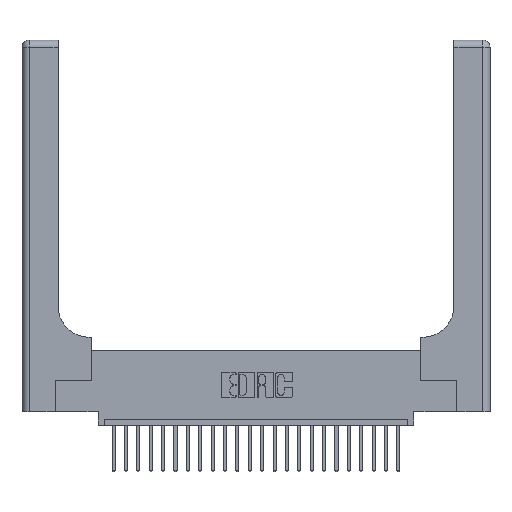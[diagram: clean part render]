
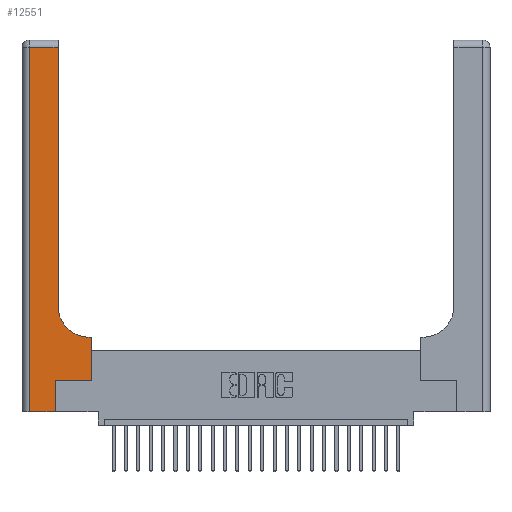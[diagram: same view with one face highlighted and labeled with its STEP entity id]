
A CAD part, top view. The second image highlights one B-rep face of the part: STEP entity #12551.
In plain terms, the highlighted planar face has unit normal (0, 0, 1).
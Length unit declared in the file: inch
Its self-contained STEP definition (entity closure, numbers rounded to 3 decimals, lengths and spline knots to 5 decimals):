
#106 = CARTESIAN_POINT ( 'NONE',  ( 0., 2.94, 0.37 ) ) ;
#196 = LINE ( 'NONE', #1382, #11151 ) ;
#1212 = EDGE_CURVE ( 'NONE', #1856, #20556, #21305, .T. ) ;
#1359 = ORIENTED_EDGE ( 'NONE', *, *, #15520, .T. ) ;
#1382 = CARTESIAN_POINT ( 'NONE',  ( 0., 0., 0.37 ) ) ;
#1856 = VERTEX_POINT ( 'NONE', #19534 ) ;
#2181 = VERTEX_POINT ( 'NONE', #15146 ) ;
#2373 = DIRECTION ( 'NONE',  ( -1., 0., 0. ) ) ;
#2596 = PLANE ( 'NONE',  #16368 ) ;
#3448 = EDGE_CURVE ( 'NONE', #17414, #22764, #19940, .T. ) ;
#3915 = LINE ( 'NONE', #106, #7043 ) ;
#5138 = ORIENTED_EDGE ( 'NONE', *, *, #19640, .T. ) ;
#5488 = DIRECTION ( 'NONE',  ( 1., 0., 0. ) ) ;
#6141 = CARTESIAN_POINT ( 'NONE',  ( 0.269, 0.25, 0.37 ) ) ;
#7043 = VECTOR ( 'NONE', #2373, 39.37008 ) ;
#7593 = DIRECTION ( 'NONE',  ( 1., 0., 0. ) ) ;
#7741 = VERTEX_POINT ( 'NONE', #16094 ) ;
#7775 = LINE ( 'NONE', #21201, #13114 ) ;
#8025 = EDGE_CURVE ( 'NONE', #21359, #1856, #20071, .T. ) ;
#8887 = EDGE_CURVE ( 'NONE', #7741, #2181, #10092, .T. ) ;
#10092 = LINE ( 'NONE', #21326, #16028 ) ;
#10170 = ORIENTED_EDGE ( 'NONE', *, *, #1212, .T. ) ;
#10438 = DIRECTION ( 'NONE',  ( 1., 0., 0. ) ) ;
#10575 = ORIENTED_EDGE ( 'NONE', *, *, #25153, .T. ) ;
#10852 = VERTEX_POINT ( 'NONE', #19851 ) ;
#11017 = VECTOR ( 'NONE', #15571, 39.37008 ) ;
#11151 = VECTOR ( 'NONE', #5488, 39.37008 ) ;
#11335 = CARTESIAN_POINT ( 'NONE',  ( 0.5585, 0.25, 0.37 ) ) ;
#11536 = CARTESIAN_POINT ( 'NONE',  ( 0.2915, 2.94, 0.37 ) ) ;
#11872 = CARTESIAN_POINT ( 'NONE',  ( 0.2915, 0.85, 0.37 ) ) ;
#12108 = CARTESIAN_POINT ( 'NONE',  ( 0.2915, 0.6, 0.37 ) ) ;
#12451 = VECTOR ( 'NONE', #16264, 39.37008 ) ;
#12551 = ADVANCED_FACE ( 'NONE', ( #18615 ), #2596, .F. ) ;
#12745 = EDGE_CURVE ( 'NONE', #2181, #21359, #196, .T. ) ;
#13114 = VECTOR ( 'NONE', #15277, 39.37008 ) ;
#13147 = AXIS2_PLACEMENT_3D ( 'NONE', #15517, #19513, #7593 ) ;
#13477 = ORIENTED_EDGE ( 'NONE', *, *, #17887, .T. ) ;
#13913 = EDGE_LOOP ( 'NONE', ( #5138, #13477, #14412, #24519, #14323, #10170, #10575, #1359, #14639 ) ) ;
#14195 = CARTESIAN_POINT ( 'NONE',  ( 0.269, 0., 0.37 ) ) ;
#14323 = ORIENTED_EDGE ( 'NONE', *, *, #8025, .T. ) ;
#14412 = ORIENTED_EDGE ( 'NONE', *, *, #8887, .T. ) ;
#14627 = CARTESIAN_POINT ( 'NONE',  ( 0., 3., 0.37 ) ) ;
#14639 = ORIENTED_EDGE ( 'NONE', *, *, #3448, .T. ) ;
#15146 = CARTESIAN_POINT ( 'NONE',  ( 0.06, 0., 0.37 ) ) ;
#15277 = DIRECTION ( 'NONE',  ( 0., 1., 0. ) ) ;
#15517 = CARTESIAN_POINT ( 'NONE',  ( 0.5415, 0.85, 0.37 ) ) ;
#15520 = EDGE_CURVE ( 'NONE', #10852, #17414, #25807, .T. ) ;
#15571 = DIRECTION ( 'NONE',  ( 0., 1., 0. ) ) ;
#16028 = VECTOR ( 'NONE', #17558, 39.37008 ) ;
#16094 = CARTESIAN_POINT ( 'NONE',  ( 0.06, 2.94, 0.37 ) ) ;
#16264 = DIRECTION ( 'NONE',  ( -1., 0., 0. ) ) ;
#16324 = VECTOR ( 'NONE', #10438, 39.37008 ) ;
#16368 = AXIS2_PLACEMENT_3D ( 'NONE', #14627, #16441, #20634 ) ;
#16441 = DIRECTION ( 'NONE',  ( 0., 0., -1. ) ) ;
#16909 = LINE ( 'NONE', #17827, #11017 ) ;
#17414 = VERTEX_POINT ( 'NONE', #20358 ) ;
#17558 = DIRECTION ( 'NONE',  ( 0., -1., 0. ) ) ;
#17827 = CARTESIAN_POINT ( 'NONE',  ( 0.2915, 3., 0.37 ) ) ;
#17887 = EDGE_CURVE ( 'NONE', #19982, #7741, #3915, .T. ) ;
#18189 = DIRECTION ( 'NONE',  ( 0., 1., 0. ) ) ;
#18615 = FACE_OUTER_BOUND ( 'NONE', #13913, .T. ) ;
#18839 = VECTOR ( 'NONE', #18189, 39.37008 ) ;
#19513 = DIRECTION ( 'NONE',  ( 0., 0., -1. ) ) ;
#19534 = CARTESIAN_POINT ( 'NONE',  ( 0.269, 0.25, 0.37 ) ) ;
#19640 = EDGE_CURVE ( 'NONE', #22764, #19982, #16909, .T. ) ;
#19851 = CARTESIAN_POINT ( 'NONE',  ( 0.5585, 0.6, 0.37 ) ) ;
#19940 = CIRCLE ( 'NONE', #13147, 0.25 ) ;
#19982 = VERTEX_POINT ( 'NONE', #11536 ) ;
#20071 = LINE ( 'NONE', #14195, #18839 ) ;
#20358 = CARTESIAN_POINT ( 'NONE',  ( 0.5415, 0.6, 0.37 ) ) ;
#20442 = CARTESIAN_POINT ( 'NONE',  ( 0.269, 0., 0.37 ) ) ;
#20556 = VERTEX_POINT ( 'NONE', #11335 ) ;
#20634 = DIRECTION ( 'NONE',  ( -1., 0., 0. ) ) ;
#21201 = CARTESIAN_POINT ( 'NONE',  ( 0.5585, 0.25, 0.37 ) ) ;
#21305 = LINE ( 'NONE', #6141, #16324 ) ;
#21326 = CARTESIAN_POINT ( 'NONE',  ( 0.06, 3., 0.37 ) ) ;
#21359 = VERTEX_POINT ( 'NONE', #20442 ) ;
#22764 = VERTEX_POINT ( 'NONE', #11872 ) ;
#24519 = ORIENTED_EDGE ( 'NONE', *, *, #12745, .T. ) ;
#25153 = EDGE_CURVE ( 'NONE', #20556, #10852, #7775, .T. ) ;
#25807 = LINE ( 'NONE', #12108, #12451 ) ;
